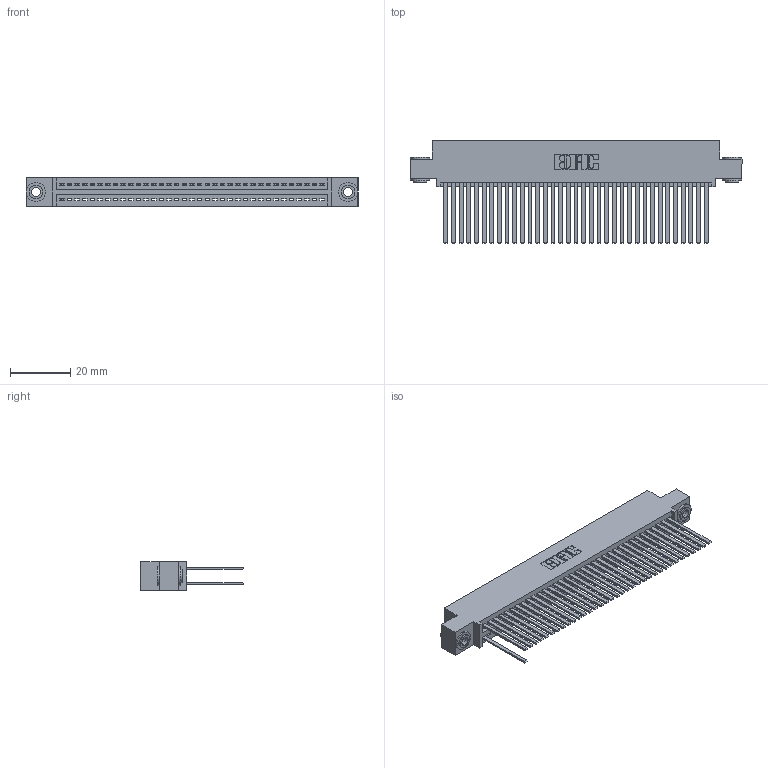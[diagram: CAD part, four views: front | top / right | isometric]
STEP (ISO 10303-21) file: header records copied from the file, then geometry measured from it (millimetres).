
FILE_DESCRIPTION (( 'STEP AP203' ), '1' );
FILE_NAME ('395-070-544-503.STEP', '2018-11-26T23:17:30', ( '' ), ( '' ), 'SwSTEP 2.0', 'SolidWorks 2016', '' );
FILE_SCHEMA (( 'CONFIG_CONTROL_DESIGN' ));
Length unit declared in the file: inch
Products named in the file (4): 345-250-002_345-250-002-102; 345-292-001_345-293-144; 345 Part_0.110 Offset - 0.156 Dia-TH; 395-070-544-503
Assembly tree (39 placements, depth 2):
  395-070-544-503
    345 Part_0.110 Offset - 0.156 Dia-TH
    345-292-001_345-293-144  x36
    345-250-002_345-250-002-102  x2
Bounding box: 110.11 x 33.96 x 9.4 mm (x, y, z)
Volume: 10775.3 mm3; surface area: 15833.1 mm2
Topology: 39 solids, 39 shells, 2024 faces, 6063 edges, 3990 vertices
Faces by surface type: plane 1376, cylinder 640, cone 8
Entity records: 27914 total; most frequent: CARTESIAN_POINT 4809, ORIENTED_EDGE 4770, DIRECTION 4239, EDGE_CURVE 2385, LINE 2093, VECTOR 2093, VERTEX_POINT 1586, AXIS2_PLACEMENT_3D 1073
